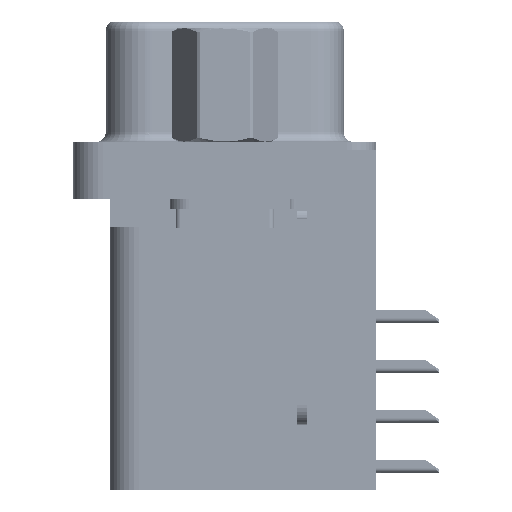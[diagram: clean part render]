
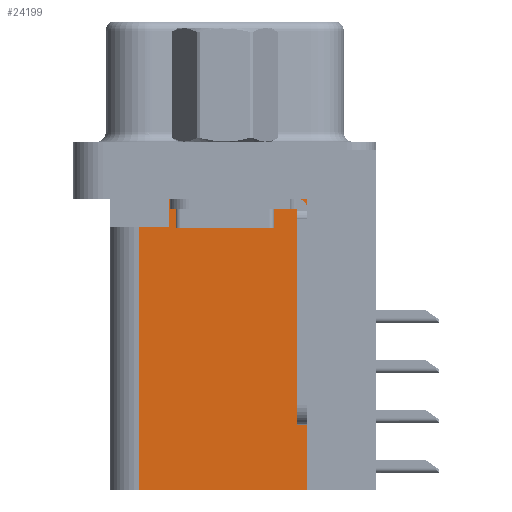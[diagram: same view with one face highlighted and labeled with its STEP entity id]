
A CAD part, left-side view. The second image highlights one B-rep face of the part: STEP entity #24199.
In plain terms, the highlighted planar face has unit normal (-1, 0, 0).
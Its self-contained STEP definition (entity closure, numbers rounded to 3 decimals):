
#1213 = EDGE_CURVE ( 'NONE', #46344, #38654, #38551, .T. ) ;
#1770 = EDGE_CURVE ( 'NONE', #45102, #4553, #41265, .T. ) ;
#3114 = DIRECTION ( 'NONE',  ( 1., 0., 0. ) ) ;
#3437 = VECTOR ( 'NONE', #11842, 1000. ) ;
#4070 = CARTESIAN_POINT ( 'NONE',  ( 3.75, -4.2, -2.5 ) ) ;
#4362 = CARTESIAN_POINT ( 'NONE',  ( 3.75, -4.2, -17.3 ) ) ;
#4553 = VERTEX_POINT ( 'NONE', #27138 ) ;
#6347 = EDGE_CURVE ( 'NONE', #38654, #11600, #35866, .T. ) ;
#6583 = VECTOR ( 'NONE', #20805, 1000. ) ;
#9250 = CARTESIAN_POINT ( 'NONE',  ( 3.75, 4.35, -17.3 ) ) ;
#10585 = VECTOR ( 'NONE', #37205, 1000. ) ;
#10685 = CARTESIAN_POINT ( 'NONE',  ( 3.75, -4.2, -2.5 ) ) ;
#10999 = VECTOR ( 'NONE', #11126, 1000. ) ;
#11126 = DIRECTION ( 'NONE',  ( 0., 1., 0. ) ) ;
#11600 = VERTEX_POINT ( 'NONE', #42465 ) ;
#11842 = DIRECTION ( 'NONE',  ( 0., 0., 1. ) ) ;
#12877 = LINE ( 'NONE', #4070, #10585 ) ;
#12963 = DIRECTION ( 'NONE',  ( 0., 0., 1. ) ) ;
#16357 = VECTOR ( 'NONE', #12963, 1000. ) ;
#17160 = CARTESIAN_POINT ( 'NONE',  ( 3.75, 0., -3.9 ) ) ;
#17832 = DIRECTION ( 'NONE',  ( 0., 0., -1. ) ) ;
#18163 = CARTESIAN_POINT ( 'NONE',  ( 3.75, 2.85, -3.9 ) ) ;
#19801 = ORIENTED_EDGE ( 'NONE', *, *, #44701, .T. ) ;
#20805 = DIRECTION ( 'NONE',  ( 0., 1., 0. ) ) ;
#23493 = FACE_OUTER_BOUND ( 'NONE', #27943, .T. ) ;
#24199 = ADVANCED_FACE ( 'NONE', ( #23493 ), #46959, .F. ) ;
#25710 = ORIENTED_EDGE ( 'NONE', *, *, #44548, .F. ) ;
#27138 = CARTESIAN_POINT ( 'NONE',  ( 3.75, 4.35, -17.3 ) ) ;
#27890 = ORIENTED_EDGE ( 'NONE', *, *, #6347, .T. ) ;
#27943 = EDGE_LOOP ( 'NONE', ( #19801, #41159, #27890, #25710, #35417, #30209 ) ) ;
#28879 = DIRECTION ( 'NONE',  ( 0., 1., 0. ) ) ;
#29449 = CARTESIAN_POINT ( 'NONE',  ( 3.75, 2.85, -3.9 ) ) ;
#30209 = ORIENTED_EDGE ( 'NONE', *, *, #34591, .T. ) ;
#31841 = CARTESIAN_POINT ( 'NONE',  ( 3.75, 2.85, -2.5 ) ) ;
#32611 = AXIS2_PLACEMENT_3D ( 'NONE', #43280, #3114, #28879 ) ;
#32863 = LINE ( 'NONE', #4362, #3437 ) ;
#34591 = EDGE_CURVE ( 'NONE', #45102, #35130, #32863, .T. ) ;
#35130 = VERTEX_POINT ( 'NONE', #10685 ) ;
#35417 = ORIENTED_EDGE ( 'NONE', *, *, #1770, .F. ) ;
#35866 = LINE ( 'NONE', #17160, #6583 ) ;
#37205 = DIRECTION ( 'NONE',  ( 0., 1., 0. ) ) ;
#37453 = VECTOR ( 'NONE', #17832, 1000. ) ;
#38551 = LINE ( 'NONE', #29449, #37453 ) ;
#38654 = VERTEX_POINT ( 'NONE', #18163 ) ;
#39194 = CARTESIAN_POINT ( 'NONE',  ( 3.75, -4.2, -17.3 ) ) ;
#41159 = ORIENTED_EDGE ( 'NONE', *, *, #1213, .T. ) ;
#41265 = LINE ( 'NONE', #42029, #10999 ) ;
#42029 = CARTESIAN_POINT ( 'NONE',  ( 3.75, -4.2, -17.3 ) ) ;
#42465 = CARTESIAN_POINT ( 'NONE',  ( 3.75, 4.35, -3.9 ) ) ;
#43280 = CARTESIAN_POINT ( 'NONE',  ( 3.75, -4.2, -17.3 ) ) ;
#44548 = EDGE_CURVE ( 'NONE', #4553, #11600, #45426, .T. ) ;
#44701 = EDGE_CURVE ( 'NONE', #35130, #46344, #12877, .T. ) ;
#45102 = VERTEX_POINT ( 'NONE', #39194 ) ;
#45426 = LINE ( 'NONE', #9250, #16357 ) ;
#46344 = VERTEX_POINT ( 'NONE', #31841 ) ;
#46959 = PLANE ( 'NONE',  #32611 ) ;
